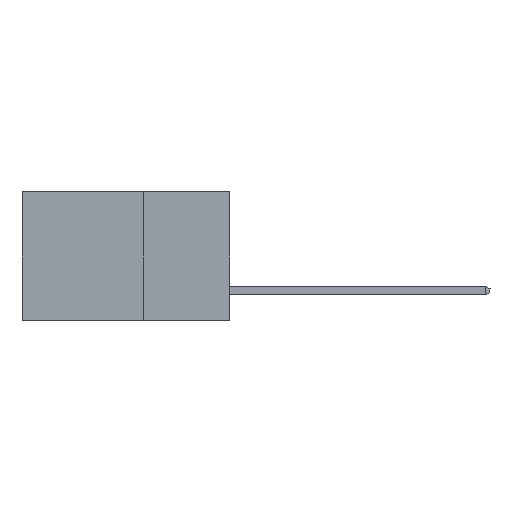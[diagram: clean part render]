
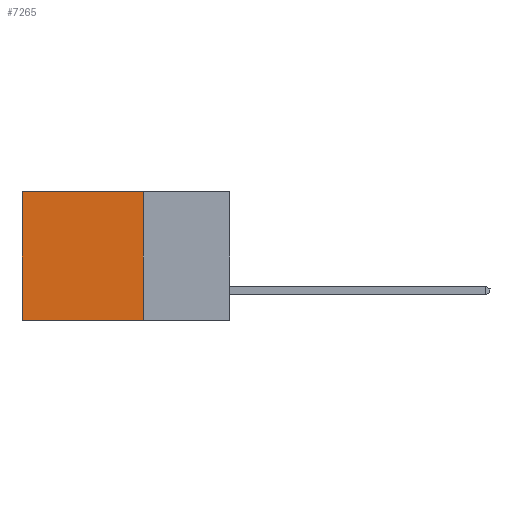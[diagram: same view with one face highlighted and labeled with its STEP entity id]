
A CAD part, left-side view. The second image highlights one B-rep face of the part: STEP entity #7265.
In plain terms, the highlighted planar face has unit normal (-1, 0, 0).
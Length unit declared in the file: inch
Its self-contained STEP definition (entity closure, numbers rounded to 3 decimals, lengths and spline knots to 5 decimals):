
#110 = DIRECTION ( 'NONE',  ( 1., 0., 0. ) ) ;
#284 = PLANE ( 'NONE',  #3121 ) ;
#635 = CARTESIAN_POINT ( 'NONE',  ( 0.2615, 0.6, -0.37 ) ) ;
#1129 = ORIENTED_EDGE ( 'NONE', *, *, #17283, .T. ) ;
#1998 = CARTESIAN_POINT ( 'NONE',  ( 0.2615, 0.25, 0. ) ) ;
#2027 = VECTOR ( 'NONE', #2374, 39.37008 ) ;
#2374 = DIRECTION ( 'NONE',  ( 0., 0., -1. ) ) ;
#2545 = EDGE_CURVE ( 'NONE', #16035, #10670, #13118, .T. ) ;
#3121 = AXIS2_PLACEMENT_3D ( 'NONE', #8572, #110, #5844 ) ;
#3175 = VECTOR ( 'NONE', #7936, 39.37008 ) ;
#3634 = CARTESIAN_POINT ( 'NONE',  ( 0.2615, 0.25, -0.37 ) ) ;
#4233 = CARTESIAN_POINT ( 'NONE',  ( 0.2615, 0.25, -0.37 ) ) ;
#4699 = EDGE_LOOP ( 'NONE', ( #17744, #17554, #12561, #1129 ) ) ;
#4948 = LINE ( 'NONE', #14971, #3175 ) ;
#5616 = CARTESIAN_POINT ( 'NONE',  ( 0.2615, 0.6, 0. ) ) ;
#5707 = VERTEX_POINT ( 'NONE', #1998 ) ;
#5844 = DIRECTION ( 'NONE',  ( 0., 0., -1. ) ) ;
#7265 = ADVANCED_FACE ( 'NONE', ( #14052 ), #284, .F. ) ;
#7936 = DIRECTION ( 'NONE',  ( 0., 1., 0. ) ) ;
#8572 = CARTESIAN_POINT ( 'NONE',  ( 0.2615, 0.25, -0.37 ) ) ;
#9017 = DIRECTION ( 'NONE',  ( 0., 0., -1. ) ) ;
#9396 = LINE ( 'NONE', #3634, #2027 ) ;
#10670 = VERTEX_POINT ( 'NONE', #12766 ) ;
#12561 = ORIENTED_EDGE ( 'NONE', *, *, #17619, .F. ) ;
#12766 = CARTESIAN_POINT ( 'NONE',  ( 0.2615, 0.6, -0.37 ) ) ;
#13118 = LINE ( 'NONE', #635, #15457 ) ;
#13580 = VECTOR ( 'NONE', #14357, 39.37008 ) ;
#14052 = FACE_OUTER_BOUND ( 'NONE', #4699, .T. ) ;
#14336 = EDGE_CURVE ( 'NONE', #17018, #10670, #17001, .T. ) ;
#14357 = DIRECTION ( 'NONE',  ( 0., 1., 0. ) ) ;
#14971 = CARTESIAN_POINT ( 'NONE',  ( 0.2615, 0.25, 0. ) ) ;
#15457 = VECTOR ( 'NONE', #9017, 39.37008 ) ;
#15616 = CARTESIAN_POINT ( 'NONE',  ( 0.2615, 0.25, -0.37 ) ) ;
#16035 = VERTEX_POINT ( 'NONE', #5616 ) ;
#17001 = LINE ( 'NONE', #4233, #13580 ) ;
#17018 = VERTEX_POINT ( 'NONE', #15616 ) ;
#17283 = EDGE_CURVE ( 'NONE', #5707, #16035, #4948, .T. ) ;
#17554 = ORIENTED_EDGE ( 'NONE', *, *, #14336, .F. ) ;
#17619 = EDGE_CURVE ( 'NONE', #5707, #17018, #9396, .T. ) ;
#17744 = ORIENTED_EDGE ( 'NONE', *, *, #2545, .T. ) ;
